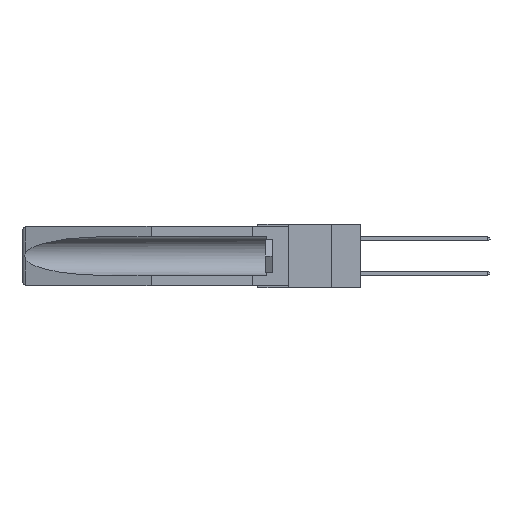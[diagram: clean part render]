
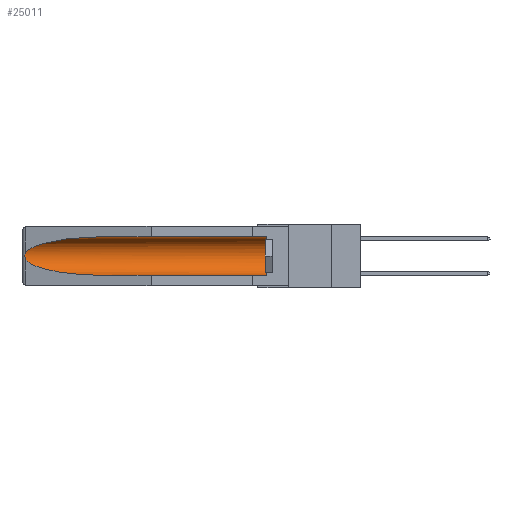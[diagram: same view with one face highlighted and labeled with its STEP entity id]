
A CAD part, left-side view. The second image highlights one B-rep face of the part: STEP entity #25011.
In plain terms, the highlighted cylindrical face has radius 2.857 mm (diameter 5.715 mm), a partial arc.
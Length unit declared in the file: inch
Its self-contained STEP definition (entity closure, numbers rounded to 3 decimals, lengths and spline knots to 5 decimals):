
#114 = EDGE_CURVE ( 'NONE', #9346, #8099, #30076, .T. ) ;
#1270 = DIRECTION ( 'NONE',  ( 0., 1., 0. ) ) ;
#1677 = CARTESIAN_POINT ( 'NONE',  ( 0.2673, 1.5327, -0.16383 ) ) ;
#2032 =( BOUNDED_CURVE ( )  B_SPLINE_CURVE ( 3, ( #31466, #26536, #12056, #6828 ),
 .UNSPECIFIED., .F., .F. ) 
 B_SPLINE_CURVE_WITH_KNOTS ( ( 4, 4 ),
 ( 4.71239, 6.08839 ),
 .UNSPECIFIED. ) 
 CURVE ( )  GEOMETRIC_REPRESENTATION_ITEM ( )  RATIONAL_B_SPLINE_CURVE ( ( 1., 0.848, 0.848, 1. ) ) 
 REPRESENTATION_ITEM ( '' )  );
#2438 = CARTESIAN_POINT ( 'NONE',  ( 0.155, 1.07973, -0.284 ) ) ;
#2835 = DIRECTION ( 'NONE',  ( 0., -1., 0. ) ) ;
#2994 = DIRECTION ( 'NONE',  ( 0., 1., 0. ) ) ;
#4054 = CARTESIAN_POINT ( 'NONE',  ( 0.26597, 1.5296, -0.19026 ) ) ;
#4464 = DIRECTION ( 'NONE',  ( 0., 1., 0. ) ) ;
#4552 = CARTESIAN_POINT ( 'NONE',  ( 0.155, 1.07973, -0.284 ) ) ;
#5616 = VERTEX_POINT ( 'NONE', #29340 ) ;
#6411 = DIRECTION ( 'NONE',  ( 0., 0., 1. ) ) ;
#6533 = CARTESIAN_POINT ( 'NONE',  ( 0.26597, 1.52961, -0.15275 ) ) ;
#6828 = CARTESIAN_POINT ( 'NONE',  ( 0.26537, 1.52718, -0.14972 ) ) ;
#8099 = VERTEX_POINT ( 'NONE', #10946 ) ;
#8931 = ORIENTED_EDGE ( 'NONE', *, *, #114, .T. ) ;
#9346 = VERTEX_POINT ( 'NONE', #15501 ) ;
#10946 = CARTESIAN_POINT ( 'NONE',  ( 0.155, 0.126, -0.059 ) ) ;
#11175 = FACE_OUTER_BOUND ( 'NONE', #31471, .T. ) ;
#11318 = CARTESIAN_POINT ( 'NONE',  ( 0.155, 1.07973, -0.059 ) ) ;
#11638 = CARTESIAN_POINT ( 'NONE',  ( 0.26537, 1.52718, -0.14972 ) ) ;
#12056 = CARTESIAN_POINT ( 'NONE',  ( 0.25451, 1.48313, -0.09465 ) ) ;
#12692 = CARTESIAN_POINT ( 'NONE',  ( 0.155, 0.126, -0.1715 ) ) ;
#12815 = VECTOR ( 'NONE', #2994, 39.37008 ) ;
#13699 = EDGE_CURVE ( 'NONE', #9346, #31641, #26993, .T. ) ;
#13824 = CARTESIAN_POINT ( 'NONE',  ( 0.2673, 1.53269, -0.17917 ) ) ;
#13920 = CARTESIAN_POINT ( 'NONE',  ( 0.26537, 1.52718, -0.19328 ) ) ;
#15103 = CARTESIAN_POINT ( 'NONE',  ( 0.155, -0.30754, -0.284 ) ) ;
#15403 =( BOUNDED_CURVE ( )  B_SPLINE_CURVE ( 3, ( #24345, #26528, #31242, #4552 ),
 .UNSPECIFIED., .F., .F. ) 
 B_SPLINE_CURVE_WITH_KNOTS ( ( 4, 4 ),
 ( 0.1948, 1.5708 ),
 .UNSPECIFIED. ) 
 CURVE ( )  GEOMETRIC_REPRESENTATION_ITEM ( )  RATIONAL_B_SPLINE_CURVE ( ( 1., 0.848, 0.848, 1. ) ) 
 REPRESENTATION_ITEM ( '' )  );
#15501 = CARTESIAN_POINT ( 'NONE',  ( 0.155, 0.126, -0.284 ) ) ;
#15532 = CARTESIAN_POINT ( 'NONE',  ( 0.155, -0.30754, -0.1715 ) ) ;
#16183 = ORIENTED_EDGE ( 'NONE', *, *, #18676, .T. ) ;
#16270 = CARTESIAN_POINT ( 'NONE',  ( 0.26655, 1.53094, -0.18657 ) ) ;
#16583 = CARTESIAN_POINT ( 'NONE',  ( 0.2675, 1.53308, -0.17534 ) ) ;
#16793 = CARTESIAN_POINT ( 'NONE',  ( 0.155, -0.30754, -0.059 ) ) ;
#16815 = VECTOR ( 'NONE', #4464, 39.37008 ) ;
#17331 = EDGE_CURVE ( 'NONE', #30264, #31121, #2032, .T. ) ;
#17637 = AXIS2_PLACEMENT_3D ( 'NONE', #12692, #2835, #25643 ) ;
#17758 = B_SPLINE_CURVE_WITH_KNOTS ( 'NONE', 3,
 ( #11638, #6533, #18835, #1677, #26120, #16583, #13824, #16270, #4054, #13920 ),
 .UNSPECIFIED., .F., .F.,
 ( 4, 2, 2, 2, 4 ),
 ( 0., 0.00029, 0.00058, 0.00087, 0.00117 ),
 .UNSPECIFIED. ) ;
#18027 = ORIENTED_EDGE ( 'NONE', *, *, #26411, .T. ) ;
#18365 = LINE ( 'NONE', #16793, #16815 ) ;
#18676 = EDGE_CURVE ( 'NONE', #5616, #31641, #15403, .T. ) ;
#18835 = CARTESIAN_POINT ( 'NONE',  ( 0.26654, 1.53092, -0.15636 ) ) ;
#20770 = CYLINDRICAL_SURFACE ( 'NONE', #28993, 0.1125 ) ;
#21977 = ORIENTED_EDGE ( 'NONE', *, *, #13699, .F. ) ;
#22587 = ORIENTED_EDGE ( 'NONE', *, *, #27842, .T. ) ;
#23363 = ORIENTED_EDGE ( 'NONE', *, *, #17331, .T. ) ;
#23817 = CARTESIAN_POINT ( 'NONE',  ( 0.26537, 1.52718, -0.14972 ) ) ;
#24345 = CARTESIAN_POINT ( 'NONE',  ( 0.26537, 1.52718, -0.19328 ) ) ;
#25011 = ADVANCED_FACE ( 'NONE', ( #11175 ), #20770, .F. ) ;
#25643 = DIRECTION ( 'NONE',  ( 0., 0., 1. ) ) ;
#26120 = CARTESIAN_POINT ( 'NONE',  ( 0.2675, 1.53308, -0.16763 ) ) ;
#26411 = EDGE_CURVE ( 'NONE', #8099, #30264, #18365, .T. ) ;
#26528 = CARTESIAN_POINT ( 'NONE',  ( 0.25451, 1.48313, -0.24835 ) ) ;
#26536 = CARTESIAN_POINT ( 'NONE',  ( 0.21114, 1.30732, -0.059 ) ) ;
#26993 = LINE ( 'NONE', #15103, #12815 ) ;
#27842 = EDGE_CURVE ( 'NONE', #31121, #5616, #17758, .T. ) ;
#28993 = AXIS2_PLACEMENT_3D ( 'NONE', #15532, #1270, #6411 ) ;
#29340 = CARTESIAN_POINT ( 'NONE',  ( 0.26537, 1.52718, -0.19328 ) ) ;
#30076 = CIRCLE ( 'NONE', #17637, 0.1125 ) ;
#30264 = VERTEX_POINT ( 'NONE', #11318 ) ;
#31121 = VERTEX_POINT ( 'NONE', #23817 ) ;
#31242 = CARTESIAN_POINT ( 'NONE',  ( 0.21114, 1.30732, -0.284 ) ) ;
#31466 = CARTESIAN_POINT ( 'NONE',  ( 0.155, 1.07973, -0.059 ) ) ;
#31471 = EDGE_LOOP ( 'NONE', ( #23363, #22587, #16183, #21977, #8931, #18027 ) ) ;
#31641 = VERTEX_POINT ( 'NONE', #2438 ) ;
